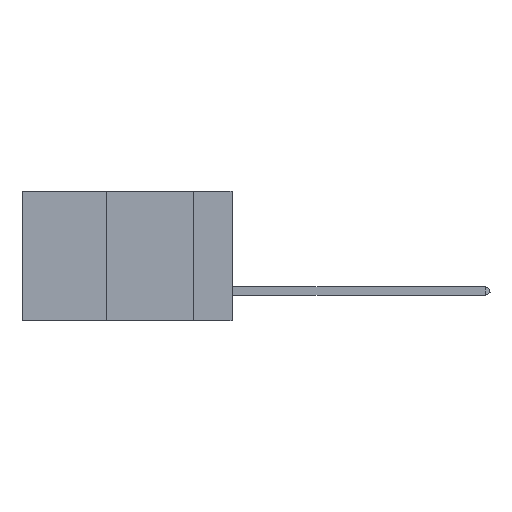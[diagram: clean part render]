
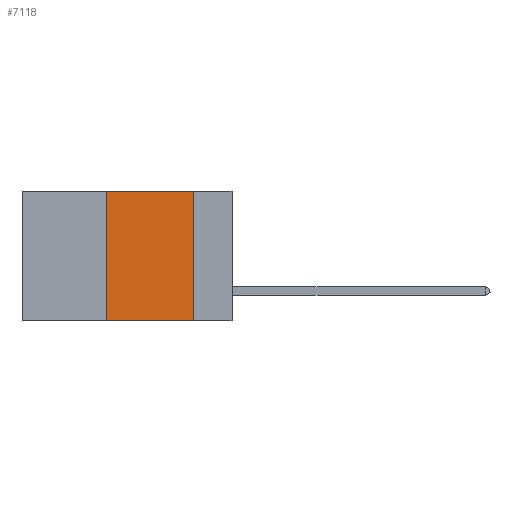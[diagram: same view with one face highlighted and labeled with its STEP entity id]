
A CAD part, left-side view. The second image highlights one B-rep face of the part: STEP entity #7118.
In plain terms, the highlighted planar face has unit normal (-1, 0, 0).
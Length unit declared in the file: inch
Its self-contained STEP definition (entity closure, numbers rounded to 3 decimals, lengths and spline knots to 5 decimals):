
#741 = DIRECTION ( 'NONE',  ( 0., -1., 0. ) ) ;
#799 = VERTEX_POINT ( 'NONE', #6126 ) ;
#1364 = LINE ( 'NONE', #14654, #2112 ) ;
#1751 = VECTOR ( 'NONE', #741, 39.37008 ) ;
#2019 = CARTESIAN_POINT ( 'NONE',  ( 0., 0.11, -0.37 ) ) ;
#2112 = VECTOR ( 'NONE', #3844, 39.37008 ) ;
#2759 = EDGE_CURVE ( 'NONE', #799, #10201, #6616, .T. ) ;
#3154 = CARTESIAN_POINT ( 'NONE',  ( 0., 0.36, 0. ) ) ;
#3439 = DIRECTION ( 'NONE',  ( 1., 0., 0. ) ) ;
#3781 = VERTEX_POINT ( 'NONE', #9328 ) ;
#3844 = DIRECTION ( 'NONE',  ( 0., 0., -1. ) ) ;
#4250 = CARTESIAN_POINT ( 'NONE',  ( 0., 0.6, 0. ) ) ;
#4398 = LINE ( 'NONE', #4250, #1751 ) ;
#6126 = CARTESIAN_POINT ( 'NONE',  ( 0., 0.36, -0.37 ) ) ;
#6224 = VECTOR ( 'NONE', #6271, 39.37008 ) ;
#6271 = DIRECTION ( 'NONE',  ( 0., -1., 0. ) ) ;
#6616 = LINE ( 'NONE', #7707, #6224 ) ;
#6845 = FACE_OUTER_BOUND ( 'NONE', #14609, .T. ) ;
#7118 = ADVANCED_FACE ( 'NONE', ( #6845 ), #13210, .F. ) ;
#7352 = EDGE_CURVE ( 'NONE', #10445, #10201, #1364, .T. ) ;
#7555 = AXIS2_PLACEMENT_3D ( 'NONE', #10877, #3439, #10763 ) ;
#7707 = CARTESIAN_POINT ( 'NONE',  ( 0., 0.6, -0.37 ) ) ;
#9328 = CARTESIAN_POINT ( 'NONE',  ( 0., 0.36, 0. ) ) ;
#10025 = VECTOR ( 'NONE', #13937, 39.37008 ) ;
#10201 = VERTEX_POINT ( 'NONE', #2019 ) ;
#10445 = VERTEX_POINT ( 'NONE', #15595 ) ;
#10575 = ORIENTED_EDGE ( 'NONE', *, *, #2759, .T. ) ;
#10763 = DIRECTION ( 'NONE',  ( 0., 0., -1. ) ) ;
#10877 = CARTESIAN_POINT ( 'NONE',  ( 0., 0.6, 0. ) ) ;
#11252 = EDGE_CURVE ( 'NONE', #3781, #10445, #4398, .T. ) ;
#11414 = ORIENTED_EDGE ( 'NONE', *, *, #7352, .F. ) ;
#11881 = ORIENTED_EDGE ( 'NONE', *, *, #11252, .F. ) ;
#13210 = PLANE ( 'NONE',  #7555 ) ;
#13852 = EDGE_CURVE ( 'NONE', #799, #3781, #15713, .T. ) ;
#13937 = DIRECTION ( 'NONE',  ( 0., 0., 1. ) ) ;
#14609 = EDGE_LOOP ( 'NONE', ( #11414, #11881, #14698, #10575 ) ) ;
#14654 = CARTESIAN_POINT ( 'NONE',  ( 0., 0.11, 0. ) ) ;
#14698 = ORIENTED_EDGE ( 'NONE', *, *, #13852, .F. ) ;
#15595 = CARTESIAN_POINT ( 'NONE',  ( 0., 0.11, 0. ) ) ;
#15713 = LINE ( 'NONE', #3154, #10025 ) ;
